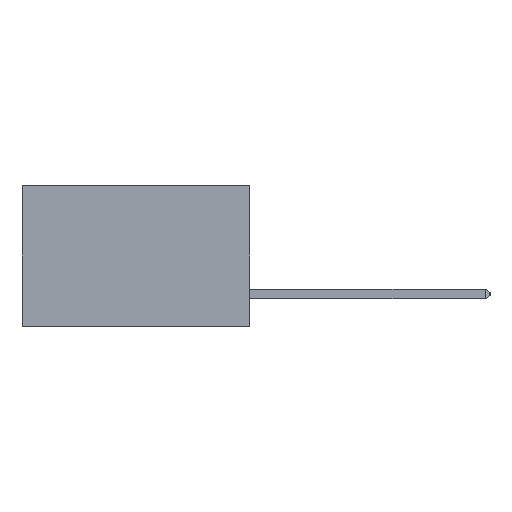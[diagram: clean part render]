
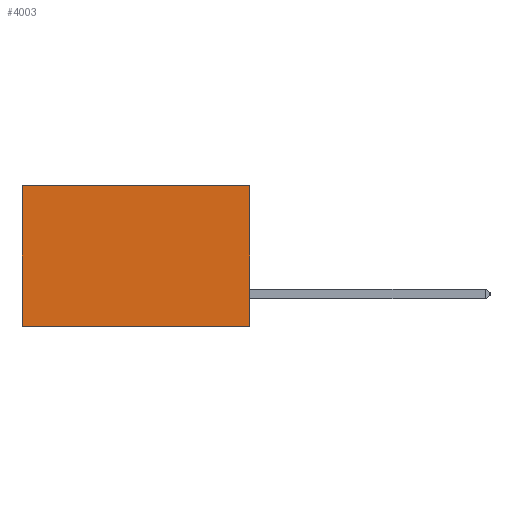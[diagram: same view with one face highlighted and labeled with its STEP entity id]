
A CAD part, left-side view. The second image highlights one B-rep face of the part: STEP entity #4003.
In plain terms, the highlighted planar face has unit normal (-1, 0, 0).
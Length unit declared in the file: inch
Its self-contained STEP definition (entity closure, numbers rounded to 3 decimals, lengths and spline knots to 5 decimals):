
#898 = CARTESIAN_POINT ( 'NONE',  ( 0.2875, 0.6, 0. ) ) ;
#927 = LINE ( 'NONE', #9129, #6929 ) ;
#1175 = EDGE_LOOP ( 'NONE', ( #4667, #28393, #2490, #16054 ) ) ;
#2490 = ORIENTED_EDGE ( 'NONE', *, *, #2960, .F. ) ;
#2960 = EDGE_CURVE ( 'NONE', #13143, #14147, #5550, .T. ) ;
#4003 = ADVANCED_FACE ( 'NONE', ( #12439 ), #21522, .F. ) ;
#4430 = DIRECTION ( 'NONE',  ( 0., 0., -1. ) ) ;
#4667 = ORIENTED_EDGE ( 'NONE', *, *, #15780, .T. ) ;
#5311 = CARTESIAN_POINT ( 'NONE',  ( 0.2875, 0., 0. ) ) ;
#5550 = LINE ( 'NONE', #21461, #22536 ) ;
#6174 = LINE ( 'NONE', #21337, #12087 ) ;
#6929 = VECTOR ( 'NONE', #13554, 39.37008 ) ;
#7214 = DIRECTION ( 'NONE',  ( 1., 0., 0. ) ) ;
#7615 = VERTEX_POINT ( 'NONE', #11726 ) ;
#9129 = CARTESIAN_POINT ( 'NONE',  ( 0.2875, 0., 0. ) ) ;
#9559 = VECTOR ( 'NONE', #10840, 39.37008 ) ;
#10840 = DIRECTION ( 'NONE',  ( 0., 1., 0. ) ) ;
#11726 = CARTESIAN_POINT ( 'NONE',  ( 0.2875, 0.6, -0.37 ) ) ;
#12087 = VECTOR ( 'NONE', #25814, 39.37008 ) ;
#12439 = FACE_OUTER_BOUND ( 'NONE', #1175, .T. ) ;
#12461 = VERTEX_POINT ( 'NONE', #898 ) ;
#13143 = VERTEX_POINT ( 'NONE', #5311 ) ;
#13428 = EDGE_CURVE ( 'NONE', #14147, #7615, #27885, .T. ) ;
#13554 = DIRECTION ( 'NONE',  ( 0., 1., 0. ) ) ;
#14147 = VERTEX_POINT ( 'NONE', #15406 ) ;
#15406 = CARTESIAN_POINT ( 'NONE',  ( 0.2875, 0., -0.37 ) ) ;
#15780 = EDGE_CURVE ( 'NONE', #12461, #7615, #6174, .T. ) ;
#16054 = ORIENTED_EDGE ( 'NONE', *, *, #21635, .T. ) ;
#17125 = DIRECTION ( 'NONE',  ( 0., 0., -1. ) ) ;
#17927 = AXIS2_PLACEMENT_3D ( 'NONE', #22464, #7214, #4430 ) ;
#21337 = CARTESIAN_POINT ( 'NONE',  ( 0.2875, 0.6, 0. ) ) ;
#21461 = CARTESIAN_POINT ( 'NONE',  ( 0.2875, 0., 0. ) ) ;
#21522 = PLANE ( 'NONE',  #17927 ) ;
#21635 = EDGE_CURVE ( 'NONE', #13143, #12461, #927, .T. ) ;
#22464 = CARTESIAN_POINT ( 'NONE',  ( 0.2875, 0., 0. ) ) ;
#22536 = VECTOR ( 'NONE', #17125, 39.37008 ) ;
#25814 = DIRECTION ( 'NONE',  ( 0., 0., -1. ) ) ;
#27885 = LINE ( 'NONE', #28437, #9559 ) ;
#28393 = ORIENTED_EDGE ( 'NONE', *, *, #13428, .F. ) ;
#28437 = CARTESIAN_POINT ( 'NONE',  ( 0.2875, 0., -0.37 ) ) ;
